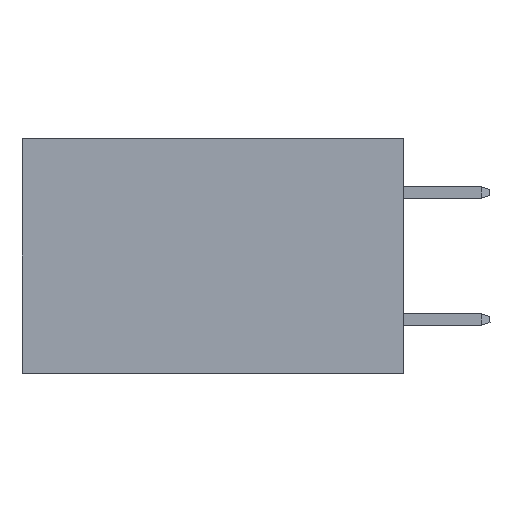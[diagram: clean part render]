
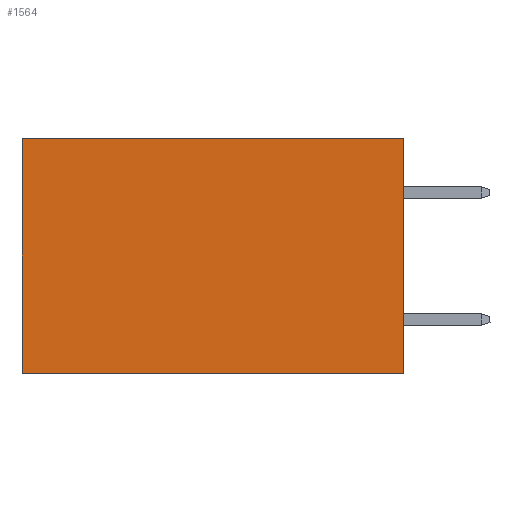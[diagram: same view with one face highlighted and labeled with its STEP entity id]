
A CAD part, left-side view. The second image highlights one B-rep face of the part: STEP entity #1564.
In plain terms, the highlighted planar face has unit normal (-1, 0, 0).
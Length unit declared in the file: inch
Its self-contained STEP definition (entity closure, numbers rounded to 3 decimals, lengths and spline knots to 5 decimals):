
#230 = FACE_OUTER_BOUND ( 'NONE', #10391, .T. ) ;
#810 = VECTOR ( 'NONE', #6598, 39.37008 ) ;
#981 = CARTESIAN_POINT ( 'NONE',  ( 0.2875, 0., 0. ) ) ;
#1180 = DIRECTION ( 'NONE',  ( 0., 1., 0. ) ) ;
#1564 = ADVANCED_FACE ( 'NONE', ( #230 ), #9709, .F. ) ;
#1569 = EDGE_CURVE ( 'NONE', #2246, #9717, #2966, .T. ) ;
#2199 = AXIS2_PLACEMENT_3D ( 'NONE', #981, #11919, #9948 ) ;
#2246 = VERTEX_POINT ( 'NONE', #8767 ) ;
#2966 = LINE ( 'NONE', #11677, #4275 ) ;
#3286 = EDGE_CURVE ( 'NONE', #9717, #5441, #11622, .T. ) ;
#3416 = ORIENTED_EDGE ( 'NONE', *, *, #1569, .F. ) ;
#3447 = EDGE_CURVE ( 'NONE', #11968, #5441, #5674, .T. ) ;
#3955 = VECTOR ( 'NONE', #7429, 39.37008 ) ;
#4275 = VECTOR ( 'NONE', #11855, 39.37008 ) ;
#4816 = CARTESIAN_POINT ( 'NONE',  ( 0.2875, 0., 0. ) ) ;
#4859 = CARTESIAN_POINT ( 'NONE',  ( 0.2875, 0., -0.37 ) ) ;
#5186 = VECTOR ( 'NONE', #1180, 39.37008 ) ;
#5441 = VERTEX_POINT ( 'NONE', #9441 ) ;
#5674 = LINE ( 'NONE', #12240, #3955 ) ;
#6163 = CARTESIAN_POINT ( 'NONE',  ( 0.2875, 0.6, 0. ) ) ;
#6429 = EDGE_CURVE ( 'NONE', #2246, #11968, #10632, .T. ) ;
#6598 = DIRECTION ( 'NONE',  ( 0., 1., 0. ) ) ;
#7244 = ORIENTED_EDGE ( 'NONE', *, *, #3286, .F. ) ;
#7249 = ORIENTED_EDGE ( 'NONE', *, *, #3447, .T. ) ;
#7269 = CARTESIAN_POINT ( 'NONE',  ( 0.2875, 0., -0.37 ) ) ;
#7429 = DIRECTION ( 'NONE',  ( 0., 0., -1. ) ) ;
#8755 = ORIENTED_EDGE ( 'NONE', *, *, #6429, .T. ) ;
#8767 = CARTESIAN_POINT ( 'NONE',  ( 0.2875, 0., 0. ) ) ;
#9441 = CARTESIAN_POINT ( 'NONE',  ( 0.2875, 0.6, -0.37 ) ) ;
#9709 = PLANE ( 'NONE',  #2199 ) ;
#9717 = VERTEX_POINT ( 'NONE', #7269 ) ;
#9948 = DIRECTION ( 'NONE',  ( 0., 0., -1. ) ) ;
#10391 = EDGE_LOOP ( 'NONE', ( #7249, #7244, #3416, #8755 ) ) ;
#10632 = LINE ( 'NONE', #4816, #810 ) ;
#11622 = LINE ( 'NONE', #4859, #5186 ) ;
#11677 = CARTESIAN_POINT ( 'NONE',  ( 0.2875, 0., 0. ) ) ;
#11855 = DIRECTION ( 'NONE',  ( 0., 0., -1. ) ) ;
#11919 = DIRECTION ( 'NONE',  ( 1., 0., 0. ) ) ;
#11968 = VERTEX_POINT ( 'NONE', #6163 ) ;
#12240 = CARTESIAN_POINT ( 'NONE',  ( 0.2875, 0.6, 0. ) ) ;
